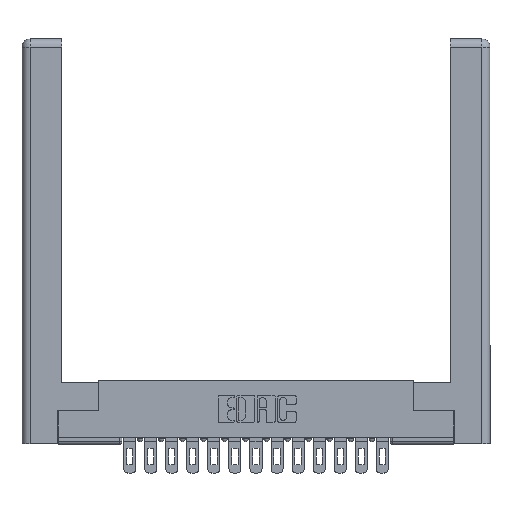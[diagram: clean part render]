
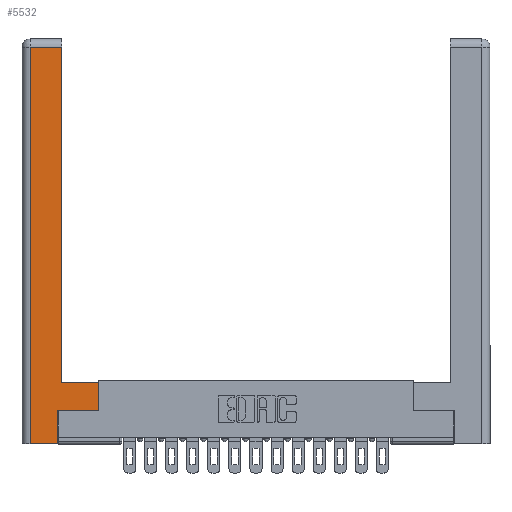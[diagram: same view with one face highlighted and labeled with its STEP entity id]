
A CAD part, top view. The second image highlights one B-rep face of the part: STEP entity #5532.
In plain terms, the highlighted planar face has unit normal (0, 0, 1).
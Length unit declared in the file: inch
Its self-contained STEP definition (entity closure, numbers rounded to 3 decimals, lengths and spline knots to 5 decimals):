
#45 = LINE ( 'NONE', #17977, #2236 ) ;
#136 = DIRECTION ( 'NONE',  ( 0., 0., -1. ) ) ;
#160 = VECTOR ( 'NONE', #15986, 39.37008 ) ;
#544 = ORIENTED_EDGE ( 'NONE', *, *, #11210, .T. ) ;
#804 = EDGE_CURVE ( 'NONE', #4055, #15623, #5738, .T. ) ;
#830 = ORIENTED_EDGE ( 'NONE', *, *, #6119, .T. ) ;
#834 = CARTESIAN_POINT ( 'NONE',  ( 0.265, 0., 0. ) ) ;
#1259 = DIRECTION ( 'NONE',  ( -1., 0., 0. ) ) ;
#1678 = LINE ( 'NONE', #6622, #16129 ) ;
#1727 = EDGE_LOOP ( 'NONE', ( #2460, #11266, #544, #13475, #830, #9945, #14113, #6463 ) ) ;
#1801 = CARTESIAN_POINT ( 'NONE',  ( 0.565, 0.45, 0. ) ) ;
#1904 = CARTESIAN_POINT ( 'NONE',  ( 0.0615, 0., 0. ) ) ;
#2236 = VECTOR ( 'NONE', #3721, 39.37008 ) ;
#2460 = ORIENTED_EDGE ( 'NONE', *, *, #804, .T. ) ;
#2638 = VERTEX_POINT ( 'NONE', #7819 ) ;
#2940 = CARTESIAN_POINT ( 'NONE',  ( 0., 0., 0. ) ) ;
#3363 = CARTESIAN_POINT ( 'NONE',  ( 0.565, 0.245, 0. ) ) ;
#3483 = DIRECTION ( 'NONE',  ( 1., 0., 0. ) ) ;
#3721 = DIRECTION ( 'NONE',  ( -1., 0., 0. ) ) ;
#3849 = VERTEX_POINT ( 'NONE', #10554 ) ;
#4055 = VERTEX_POINT ( 'NONE', #16655 ) ;
#5532 = ADVANCED_FACE ( 'NONE', ( #15690 ), #16905, .F. ) ;
#5738 = LINE ( 'NONE', #7757, #8552 ) ;
#6033 = VECTOR ( 'NONE', #14389, 39.37008 ) ;
#6119 = EDGE_CURVE ( 'NONE', #8225, #3849, #6447, .T. ) ;
#6398 = VECTOR ( 'NONE', #3483, 39.37008 ) ;
#6403 = CARTESIAN_POINT ( 'NONE',  ( 0.265, 0., 0. ) ) ;
#6447 = LINE ( 'NONE', #7601, #11721 ) ;
#6463 = ORIENTED_EDGE ( 'NONE', *, *, #8445, .T. ) ;
#6622 = CARTESIAN_POINT ( 'NONE',  ( 0.0615, 2.94, 0. ) ) ;
#7601 = CARTESIAN_POINT ( 'NONE',  ( 0.265, 0.245, 0. ) ) ;
#7757 = CARTESIAN_POINT ( 'NONE',  ( 0.295, 3., 0. ) ) ;
#7819 = CARTESIAN_POINT ( 'NONE',  ( 0.0615, 2.94, 0. ) ) ;
#8199 = VERTEX_POINT ( 'NONE', #11604 ) ;
#8225 = VERTEX_POINT ( 'NONE', #834 ) ;
#8445 = EDGE_CURVE ( 'NONE', #14403, #4055, #45, .T. ) ;
#8542 = DIRECTION ( 'NONE',  ( -1., 0., 0. ) ) ;
#8552 = VECTOR ( 'NONE', #10565, 39.37008 ) ;
#9287 = LINE ( 'NONE', #1801, #6033 ) ;
#9862 = CARTESIAN_POINT ( 'NONE',  ( 0.565, 0.245, 0. ) ) ;
#9945 = ORIENTED_EDGE ( 'NONE', *, *, #13359, .T. ) ;
#10119 = LINE ( 'NONE', #3363, #6398 ) ;
#10134 = DIRECTION ( 'NONE',  ( 0., -1., 0. ) ) ;
#10554 = CARTESIAN_POINT ( 'NONE',  ( 0.265, 0.245, 0. ) ) ;
#10565 = DIRECTION ( 'NONE',  ( 0., 1., 0. ) ) ;
#11210 = EDGE_CURVE ( 'NONE', #2638, #8199, #12141, .T. ) ;
#11266 = ORIENTED_EDGE ( 'NONE', *, *, #17378, .T. ) ;
#11604 = CARTESIAN_POINT ( 'NONE',  ( 0.0615, 0., 0. ) ) ;
#11721 = VECTOR ( 'NONE', #14685, 39.37008 ) ;
#12141 = LINE ( 'NONE', #1904, #13231 ) ;
#12323 = CARTESIAN_POINT ( 'NONE',  ( 0.295, 2.94, 0. ) ) ;
#13231 = VECTOR ( 'NONE', #10134, 39.37008 ) ;
#13359 = EDGE_CURVE ( 'NONE', #3849, #17472, #10119, .T. ) ;
#13475 = ORIENTED_EDGE ( 'NONE', *, *, #16560, .T. ) ;
#14113 = ORIENTED_EDGE ( 'NONE', *, *, #17632, .T. ) ;
#14153 = LINE ( 'NONE', #6403, #160 ) ;
#14389 = DIRECTION ( 'NONE',  ( 0., 1., 0. ) ) ;
#14403 = VERTEX_POINT ( 'NONE', #15312 ) ;
#14685 = DIRECTION ( 'NONE',  ( 0., 1., 0. ) ) ;
#15312 = CARTESIAN_POINT ( 'NONE',  ( 0.565, 0.45, 0. ) ) ;
#15423 = AXIS2_PLACEMENT_3D ( 'NONE', #2940, #136, #8542 ) ;
#15623 = VERTEX_POINT ( 'NONE', #12323 ) ;
#15690 = FACE_OUTER_BOUND ( 'NONE', #1727, .T. ) ;
#15986 = DIRECTION ( 'NONE',  ( 1., 0., 0. ) ) ;
#16129 = VECTOR ( 'NONE', #1259, 39.37008 ) ;
#16560 = EDGE_CURVE ( 'NONE', #8199, #8225, #14153, .T. ) ;
#16655 = CARTESIAN_POINT ( 'NONE',  ( 0.295, 0.45, 0. ) ) ;
#16905 = PLANE ( 'NONE',  #15423 ) ;
#17378 = EDGE_CURVE ( 'NONE', #15623, #2638, #1678, .T. ) ;
#17472 = VERTEX_POINT ( 'NONE', #9862 ) ;
#17632 = EDGE_CURVE ( 'NONE', #17472, #14403, #9287, .T. ) ;
#17977 = CARTESIAN_POINT ( 'NONE',  ( 0.295, 0.45, 0. ) ) ;
